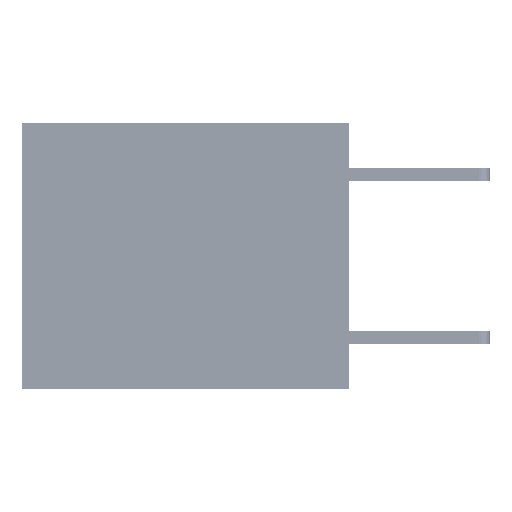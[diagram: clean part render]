
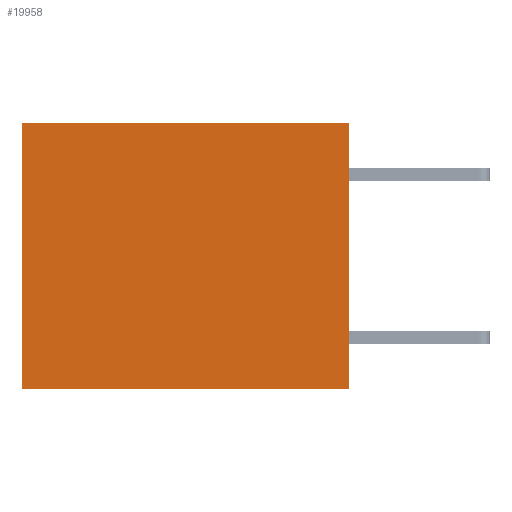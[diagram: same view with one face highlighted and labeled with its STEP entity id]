
A CAD part, left-side view. The second image highlights one B-rep face of the part: STEP entity #19958.
In plain terms, the highlighted planar face has unit normal (-1, 0, 0).
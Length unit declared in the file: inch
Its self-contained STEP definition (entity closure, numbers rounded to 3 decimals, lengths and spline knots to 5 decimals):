
#3013 = EDGE_CURVE ( 'NONE', #12729, #5447, #17056, .T. ) ;
#5383 = VECTOR ( 'NONE', #5735, 39.37008 ) ;
#5447 = VERTEX_POINT ( 'NONE', #24244 ) ;
#5735 = DIRECTION ( 'NONE',  ( 0., 1., 0. ) ) ;
#6900 = VECTOR ( 'NONE', #31418, 39.37008 ) ;
#9212 = CARTESIAN_POINT ( 'NONE',  ( 0.3165, 0., -0.49 ) ) ;
#9921 = ORIENTED_EDGE ( 'NONE', *, *, #34029, .F. ) ;
#10130 = CARTESIAN_POINT ( 'NONE',  ( 0.3165, 0.6, 0. ) ) ;
#11409 = PLANE ( 'NONE',  #19974 ) ;
#12137 = DIRECTION ( 'NONE',  ( 0., 0., -1. ) ) ;
#12242 = CARTESIAN_POINT ( 'NONE',  ( 0.3165, 0.6, -0.49 ) ) ;
#12305 = LINE ( 'NONE', #31190, #6900 ) ;
#12729 = VERTEX_POINT ( 'NONE', #10130 ) ;
#16501 = LINE ( 'NONE', #33476, #23550 ) ;
#17056 = LINE ( 'NONE', #12242, #19588 ) ;
#17104 = CARTESIAN_POINT ( 'NONE',  ( 0.3165, 0., 0. ) ) ;
#17234 = DIRECTION ( 'NONE',  ( 0., 0., -1. ) ) ;
#19588 = VECTOR ( 'NONE', #12137, 39.37008 ) ;
#19958 = ADVANCED_FACE ( 'NONE', ( #21229 ), #11409, .F. ) ;
#19974 = AXIS2_PLACEMENT_3D ( 'NONE', #9212, #26723, #17234 ) ;
#20289 = DIRECTION ( 'NONE',  ( 0., 0., -1. ) ) ;
#20770 = LINE ( 'NONE', #32323, #5383 ) ;
#21229 = FACE_OUTER_BOUND ( 'NONE', #33520, .T. ) ;
#21726 = EDGE_CURVE ( 'NONE', #28855, #31451, #16501, .T. ) ;
#23415 = CARTESIAN_POINT ( 'NONE',  ( 0.3165, 0., -0.49 ) ) ;
#23550 = VECTOR ( 'NONE', #20289, 39.37008 ) ;
#24244 = CARTESIAN_POINT ( 'NONE',  ( 0.3165, 0.6, -0.49 ) ) ;
#26723 = DIRECTION ( 'NONE',  ( 1., 0., 0. ) ) ;
#27064 = ORIENTED_EDGE ( 'NONE', *, *, #30806, .T. ) ;
#28855 = VERTEX_POINT ( 'NONE', #17104 ) ;
#30806 = EDGE_CURVE ( 'NONE', #28855, #12729, #12305, .T. ) ;
#31190 = CARTESIAN_POINT ( 'NONE',  ( 0.3165, 0., 0. ) ) ;
#31418 = DIRECTION ( 'NONE',  ( 0., 1., 0. ) ) ;
#31451 = VERTEX_POINT ( 'NONE', #23415 ) ;
#32323 = CARTESIAN_POINT ( 'NONE',  ( 0.3165, 0., -0.49 ) ) ;
#32396 = ORIENTED_EDGE ( 'NONE', *, *, #21726, .F. ) ;
#33476 = CARTESIAN_POINT ( 'NONE',  ( 0.3165, 0., -0.49 ) ) ;
#33520 = EDGE_LOOP ( 'NONE', ( #33900, #9921, #32396, #27064 ) ) ;
#33900 = ORIENTED_EDGE ( 'NONE', *, *, #3013, .T. ) ;
#34029 = EDGE_CURVE ( 'NONE', #31451, #5447, #20770, .T. ) ;
